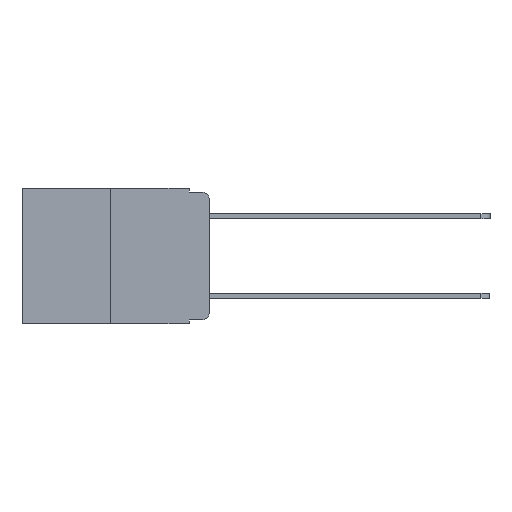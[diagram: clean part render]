
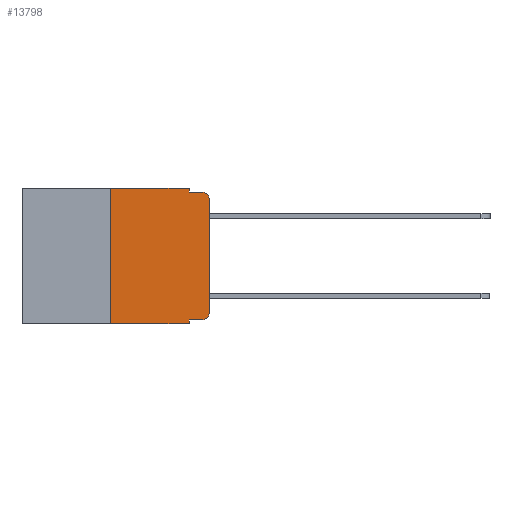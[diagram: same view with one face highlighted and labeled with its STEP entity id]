
A CAD part, left-side view. The second image highlights one B-rep face of the part: STEP entity #13798.
In plain terms, the highlighted planar face has unit normal (-1, 0, 0).
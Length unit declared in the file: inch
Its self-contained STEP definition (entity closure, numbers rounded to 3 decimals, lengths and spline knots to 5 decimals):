
#561 = CARTESIAN_POINT ( 'NONE',  ( 0., 0., -0.03 ) ) ;
#612 = EDGE_CURVE ( 'NONE', #16335, #23368, #21473, .T. ) ;
#1100 = EDGE_CURVE ( 'NONE', #23368, #1532, #21446, .T. ) ;
#1532 = VERTEX_POINT ( 'NONE', #5991 ) ;
#1622 = DIRECTION ( 'NONE',  ( 0., -1., 0. ) ) ;
#1915 = VERTEX_POINT ( 'NONE', #561 ) ;
#2003 = EDGE_LOOP ( 'NONE', ( #4772, #5934, #23373, #6749, #16907, #18954, #16170, #17145, #24078, #9893 ) ) ;
#2080 = VECTOR ( 'NONE', #6568, 39.37008 ) ;
#2274 = VERTEX_POINT ( 'NONE', #23902 ) ;
#3039 = VERTEX_POINT ( 'NONE', #19836 ) ;
#3240 = FACE_OUTER_BOUND ( 'NONE', #2003, .T. ) ;
#4432 = CIRCLE ( 'NONE', #13338, 0.02 ) ;
#4524 = CARTESIAN_POINT ( 'NONE',  ( 0., 0.02, -0.333 ) ) ;
#4772 = ORIENTED_EDGE ( 'NONE', *, *, #21215, .T. ) ;
#5084 = LINE ( 'NONE', #19139, #14707 ) ;
#5457 = CARTESIAN_POINT ( 'NONE',  ( 0., 0.051, 0. ) ) ;
#5934 = ORIENTED_EDGE ( 'NONE', *, *, #6861, .T. ) ;
#5991 = CARTESIAN_POINT ( 'NONE',  ( 0., 0.02, -0.01 ) ) ;
#6102 = VECTOR ( 'NONE', #18568, 39.37008 ) ;
#6458 = CARTESIAN_POINT ( 'NONE',  ( 0., 0., 0. ) ) ;
#6568 = DIRECTION ( 'NONE',  ( 0., -1., 0. ) ) ;
#6581 = AXIS2_PLACEMENT_3D ( 'NONE', #7571, #20872, #9501 ) ;
#6600 = DIRECTION ( 'NONE',  ( 0., -1., 0. ) ) ;
#6749 = ORIENTED_EDGE ( 'NONE', *, *, #612, .F. ) ;
#6855 = CARTESIAN_POINT ( 'NONE',  ( 0., 0.051, -0.343 ) ) ;
#6861 = EDGE_CURVE ( 'NONE', #1915, #1532, #10030, .T. ) ;
#7239 = DIRECTION ( 'NONE',  ( 0., 0., 1. ) ) ;
#7477 = LINE ( 'NONE', #12300, #2080 ) ;
#7556 = EDGE_CURVE ( 'NONE', #21244, #3039, #4432, .T. ) ;
#7571 = CARTESIAN_POINT ( 'NONE',  ( 0., 0.02, -0.03 ) ) ;
#7718 = DIRECTION ( 'NONE',  ( 0., 0., -1. ) ) ;
#8253 = DIRECTION ( 'NONE',  ( 0., -1., 0. ) ) ;
#9012 = PLANE ( 'NONE',  #17792 ) ;
#9501 = DIRECTION ( 'NONE',  ( 0., 0., -1. ) ) ;
#9893 = ORIENTED_EDGE ( 'NONE', *, *, #7556, .T. ) ;
#10030 = CIRCLE ( 'NONE', #6581, 0.02 ) ;
#11366 = VECTOR ( 'NONE', #7718, 39.37008 ) ;
#11457 = DIRECTION ( 'NONE',  ( -1., 0., 0. ) ) ;
#12257 = CARTESIAN_POINT ( 'NONE',  ( 0., 0.051, 0. ) ) ;
#12300 = CARTESIAN_POINT ( 'NONE',  ( 0., 0.051, -0.333 ) ) ;
#12451 = LINE ( 'NONE', #16728, #6102 ) ;
#12825 = DIRECTION ( 'NONE',  ( 0., 0., -1. ) ) ;
#13289 = LINE ( 'NONE', #20567, #22806 ) ;
#13338 = AXIS2_PLACEMENT_3D ( 'NONE', #22819, #11457, #24688 ) ;
#13798 = ADVANCED_FACE ( 'NONE', ( #3240 ), #9012, .F. ) ;
#14707 = VECTOR ( 'NONE', #1622, 39.37008 ) ;
#15970 = CARTESIAN_POINT ( 'NONE',  ( 0., 0.25, 0. ) ) ;
#16158 = LINE ( 'NONE', #18081, #21189 ) ;
#16170 = ORIENTED_EDGE ( 'NONE', *, *, #18935, .T. ) ;
#16274 = EDGE_CURVE ( 'NONE', #2274, #21955, #12451, .T. ) ;
#16335 = VERTEX_POINT ( 'NONE', #5457 ) ;
#16412 = VECTOR ( 'NONE', #8253, 39.37008 ) ;
#16728 = CARTESIAN_POINT ( 'NONE',  ( 0., 0.051, 0. ) ) ;
#16907 = ORIENTED_EDGE ( 'NONE', *, *, #19997, .F. ) ;
#17145 = ORIENTED_EDGE ( 'NONE', *, *, #16274, .F. ) ;
#17516 = CARTESIAN_POINT ( 'NONE',  ( 0., 0.051, -0.01 ) ) ;
#17792 = AXIS2_PLACEMENT_3D ( 'NONE', #18504, #24160, #12825 ) ;
#18081 = CARTESIAN_POINT ( 'NONE',  ( 0., 0.473, 0. ) ) ;
#18478 = VECTOR ( 'NONE', #19845, 39.37008 ) ;
#18504 = CARTESIAN_POINT ( 'NONE',  ( 0., 0.473, 0. ) ) ;
#18568 = DIRECTION ( 'NONE',  ( 0., 0., -1. ) ) ;
#18935 = EDGE_CURVE ( 'NONE', #22529, #21955, #5084, .T. ) ;
#18954 = ORIENTED_EDGE ( 'NONE', *, *, #24148, .F. ) ;
#19139 = CARTESIAN_POINT ( 'NONE',  ( 0., 0.473, -0.343 ) ) ;
#19151 = VERTEX_POINT ( 'NONE', #15970 ) ;
#19836 = CARTESIAN_POINT ( 'NONE',  ( 0., 0., -0.313 ) ) ;
#19845 = DIRECTION ( 'NONE',  ( 0., 0., 1. ) ) ;
#19997 = EDGE_CURVE ( 'NONE', #19151, #16335, #16158, .T. ) ;
#20567 = CARTESIAN_POINT ( 'NONE',  ( 0., 0.25, 0. ) ) ;
#20609 = EDGE_CURVE ( 'NONE', #2274, #21244, #7477, .T. ) ;
#20872 = DIRECTION ( 'NONE',  ( -1., 0., 0. ) ) ;
#21189 = VECTOR ( 'NONE', #6600, 39.37008 ) ;
#21215 = EDGE_CURVE ( 'NONE', #3039, #1915, #23479, .T. ) ;
#21244 = VERTEX_POINT ( 'NONE', #4524 ) ;
#21446 = LINE ( 'NONE', #17516, #16412 ) ;
#21473 = LINE ( 'NONE', #12257, #11366 ) ;
#21928 = CARTESIAN_POINT ( 'NONE',  ( 0., 0.051, -0.01 ) ) ;
#21955 = VERTEX_POINT ( 'NONE', #6855 ) ;
#22529 = VERTEX_POINT ( 'NONE', #23030 ) ;
#22806 = VECTOR ( 'NONE', #7239, 39.37008 ) ;
#22819 = CARTESIAN_POINT ( 'NONE',  ( 0., 0.02, -0.313 ) ) ;
#23030 = CARTESIAN_POINT ( 'NONE',  ( 0., 0.25, -0.343 ) ) ;
#23368 = VERTEX_POINT ( 'NONE', #21928 ) ;
#23373 = ORIENTED_EDGE ( 'NONE', *, *, #1100, .F. ) ;
#23479 = LINE ( 'NONE', #6458, #18478 ) ;
#23902 = CARTESIAN_POINT ( 'NONE',  ( 0., 0.051, -0.333 ) ) ;
#24078 = ORIENTED_EDGE ( 'NONE', *, *, #20609, .T. ) ;
#24148 = EDGE_CURVE ( 'NONE', #22529, #19151, #13289, .T. ) ;
#24160 = DIRECTION ( 'NONE',  ( 1., 0., 0. ) ) ;
#24688 = DIRECTION ( 'NONE',  ( 0., 0., -1. ) ) ;
